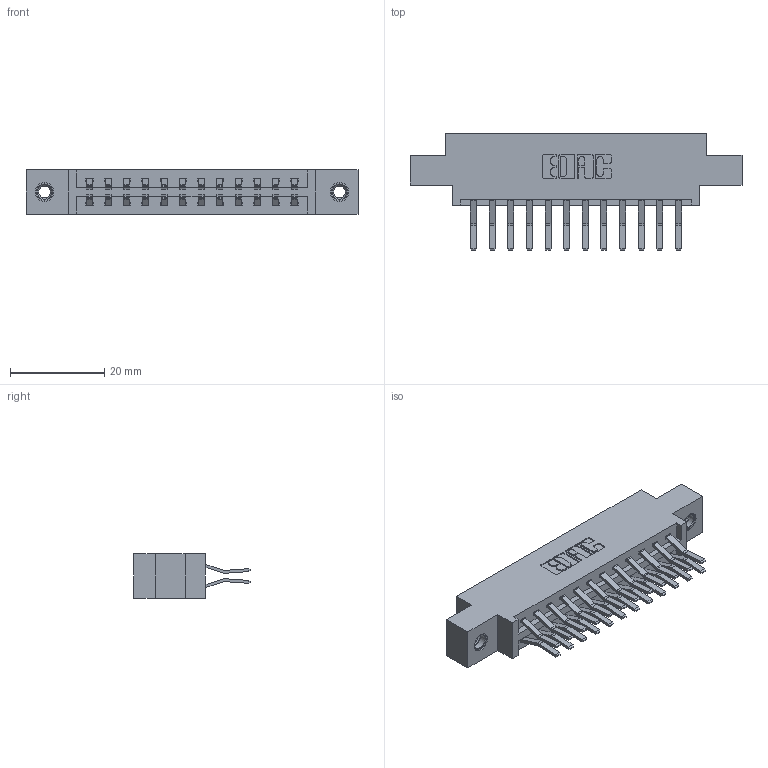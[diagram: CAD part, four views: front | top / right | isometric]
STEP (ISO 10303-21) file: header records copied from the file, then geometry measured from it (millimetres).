
FILE_DESCRIPTION (( 'STEP AP203' ), '1' );
FILE_NAME ('337-024-560-807.STEP', '2019-10-10T21:23:16', ( '' ), ( '' ), 'SwSTEP 2.0', 'SolidWorks 2016', '' );
FILE_SCHEMA (( 'CONFIG_CONTROL_DESIGN' ));
Length unit declared in the file: inch
Products named in the file (4): 345-292-001_560 Tail; 345-250-001_345-250-005-103; 337 Part_0.170 Offset - 0.156 Dia-TI; 337-024-560-807
Assembly tree (27 placements, depth 2):
  337-024-560-807
    337 Part_0.170 Offset - 0.156 Dia-TI
    345-292-001_560 Tail  x24
    345-250-001_345-250-005-103  x2
Bounding box: 70.56 x 24.78 x 9.4 mm (x, y, z)
Volume: 7063.3 mm3; surface area: 8292.7 mm2
Topology: 27 solids, 27 shells, 1522 faces, 4467 edges, 2938 vertices
Faces by surface type: plane 1018, cylinder 488, cone 12, torus 4
Entity records: 14590 total; most frequent: CARTESIAN_POINT 2465, ORIENTED_EDGE 2394, DIRECTION 2187, EDGE_CURVE 1197, VECTOR 1045, LINE 1045, VERTEX_POINT 792, AXIS2_PLACEMENT_3D 571
